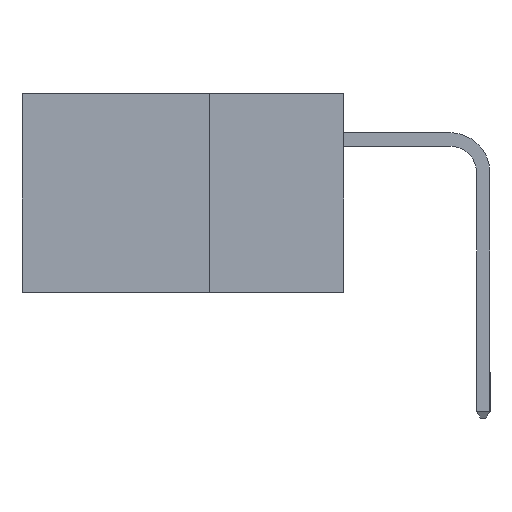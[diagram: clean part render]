
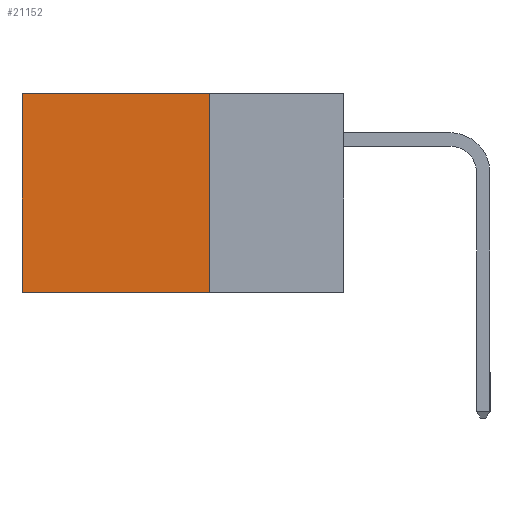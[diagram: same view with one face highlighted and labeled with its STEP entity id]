
A CAD part, left-side view. The second image highlights one B-rep face of the part: STEP entity #21152.
In plain terms, the highlighted planar face has unit normal (-1, 0, 0).
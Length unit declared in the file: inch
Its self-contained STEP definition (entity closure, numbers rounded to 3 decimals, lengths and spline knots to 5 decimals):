
#804 = LINE ( 'NONE', #25139, #6318 ) ;
#1085 = CARTESIAN_POINT ( 'NONE',  ( 0.298, 0.25, 0. ) ) ;
#3825 = LINE ( 'NONE', #5917, #24139 ) ;
#4173 = VERTEX_POINT ( 'NONE', #11255 ) ;
#4484 = VERTEX_POINT ( 'NONE', #19423 ) ;
#5286 = CARTESIAN_POINT ( 'NONE',  ( 0.298, 0.25, 0. ) ) ;
#5801 = PLANE ( 'NONE',  #11904 ) ;
#5917 = CARTESIAN_POINT ( 'NONE',  ( 0.298, 0.25, 0. ) ) ;
#6318 = VECTOR ( 'NONE', #20203, 39.37008 ) ;
#6990 = ORIENTED_EDGE ( 'NONE', *, *, #25323, .F. ) ;
#7403 = CARTESIAN_POINT ( 'NONE',  ( 0.298, 0.6, 0. ) ) ;
#8140 = DIRECTION ( 'NONE',  ( 1., 0., 0. ) ) ;
#8779 = LINE ( 'NONE', #5286, #22165 ) ;
#9673 = DIRECTION ( 'NONE',  ( 0., 1., 0. ) ) ;
#10257 = DIRECTION ( 'NONE',  ( 0., 0., -1. ) ) ;
#10468 = DIRECTION ( 'NONE',  ( 0., 0., -1. ) ) ;
#11255 = CARTESIAN_POINT ( 'NONE',  ( 0.298, 0.6, -0.37 ) ) ;
#11904 = AXIS2_PLACEMENT_3D ( 'NONE', #1085, #8140, #10468 ) ;
#11906 = EDGE_CURVE ( 'NONE', #4484, #28393, #8779, .T. ) ;
#13013 = DIRECTION ( 'NONE',  ( 0., 0., -1. ) ) ;
#13521 = ORIENTED_EDGE ( 'NONE', *, *, #11906, .T. ) ;
#15618 = LINE ( 'NONE', #7403, #29356 ) ;
#15758 = ORIENTED_EDGE ( 'NONE', *, *, #21012, .T. ) ;
#18338 = ORIENTED_EDGE ( 'NONE', *, *, #27906, .F. ) ;
#18744 = EDGE_LOOP ( 'NONE', ( #15758, #6990, #18338, #13521 ) ) ;
#19135 = CARTESIAN_POINT ( 'NONE',  ( 0.298, 0.6, 0. ) ) ;
#19423 = CARTESIAN_POINT ( 'NONE',  ( 0.298, 0.25, 0. ) ) ;
#20203 = DIRECTION ( 'NONE',  ( 0., 1., 0. ) ) ;
#21012 = EDGE_CURVE ( 'NONE', #28393, #4173, #15618, .T. ) ;
#21152 = ADVANCED_FACE ( 'NONE', ( #23952 ), #5801, .F. ) ;
#22165 = VECTOR ( 'NONE', #9673, 39.37008 ) ;
#23952 = FACE_OUTER_BOUND ( 'NONE', #18744, .T. ) ;
#24139 = VECTOR ( 'NONE', #13013, 39.37008 ) ;
#25139 = CARTESIAN_POINT ( 'NONE',  ( 0.298, 0.25, -0.37 ) ) ;
#25255 = VERTEX_POINT ( 'NONE', #29491 ) ;
#25323 = EDGE_CURVE ( 'NONE', #25255, #4173, #804, .T. ) ;
#27906 = EDGE_CURVE ( 'NONE', #4484, #25255, #3825, .T. ) ;
#28393 = VERTEX_POINT ( 'NONE', #19135 ) ;
#29356 = VECTOR ( 'NONE', #10257, 39.37008 ) ;
#29491 = CARTESIAN_POINT ( 'NONE',  ( 0.298, 0.25, -0.37 ) ) ;
